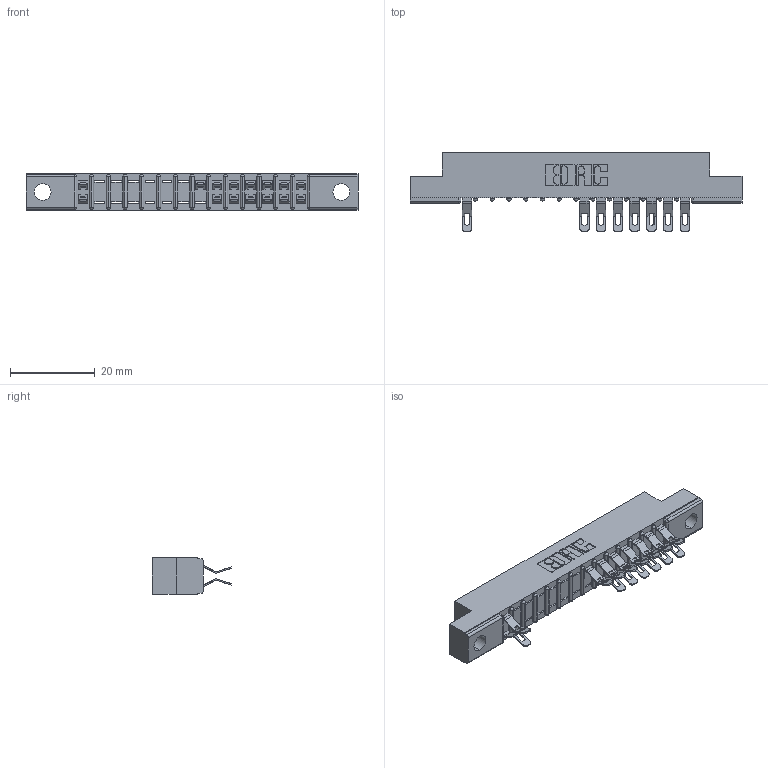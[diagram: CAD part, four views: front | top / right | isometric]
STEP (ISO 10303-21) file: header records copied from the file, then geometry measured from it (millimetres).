
FILE_DESCRIPTION (( 'STEP AP203' ), '1' );
FILE_NAME ('307-028-555-204.STEP', '2018-08-04T17:00:29', ( '' ), ( '' ), 'SwSTEP 2.0', 'SolidWorks 2016', '' );
FILE_SCHEMA (( 'CONFIG_CONTROL_DESIGN' ));
Length unit declared in the file: inch
Products named in the file (3): 307-028-555-204; 307 Part_.156 Dia Mounting Holes; 307-290-001_555
Assembly tree (16 placements, depth 2):
  307-028-555-204
    307 Part_.156 Dia Mounting Holes
    307-290-001_555  x15
Bounding box: 78.49 x 18.75 x 8.71 mm (x, y, z)
Volume: 4905.1 mm3; surface area: 7387.8 mm2
Topology: 16 solids, 16 shells, 1192 faces, 3490 edges, 2264 vertices
Faces by surface type: plane 672, cylinder 490, sphere 30
Entity records: 16441 total; most frequent: CARTESIAN_POINT 2763, ORIENTED_EDGE 2748, DIRECTION 2704, EDGE_CURVE 1374, LINE 1038, VECTOR 1038, VERTEX_POINT 892, AXIS2_PLACEMENT_3D 833
